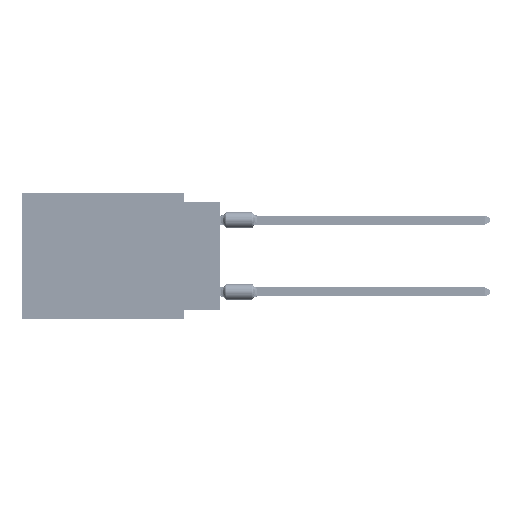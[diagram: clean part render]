
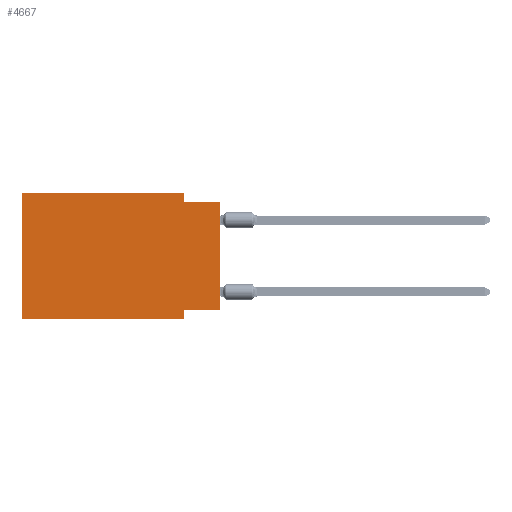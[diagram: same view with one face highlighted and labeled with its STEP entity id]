
A CAD part, left-side view. The second image highlights one B-rep face of the part: STEP entity #4667.
In plain terms, the highlighted planar face has unit normal (-1, 0, 0).
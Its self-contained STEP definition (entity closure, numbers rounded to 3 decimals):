
#9 = ORIENTED_EDGE ( 'NONE', *, *, #9248, .F. ) ;
#774 = CARTESIAN_POINT ( 'NONE',  ( 0., 0., -0.635 ) ) ;
#1195 = ORIENTED_EDGE ( 'NONE', *, *, #63471, .T. ) ;
#1686 = VECTOR ( 'NONE', #52025, 1000. ) ;
#3963 = FACE_OUTER_BOUND ( 'NONE', #36349, .T. ) ;
#4667 = ADVANCED_FACE ( 'NONE', ( #3963 ), #26721, .F. ) ;
#5052 = VECTOR ( 'NONE', #40132, 1000. ) ;
#9248 = EDGE_CURVE ( 'NONE', #35094, #36176, #18670, .T. ) ;
#10494 = CARTESIAN_POINT ( 'NONE',  ( 0., 2.54, 0. ) ) ;
#11138 = VERTEX_POINT ( 'NONE', #43943 ) ;
#11464 = ORIENTED_EDGE ( 'NONE', *, *, #60808, .T. ) ;
#11735 = CARTESIAN_POINT ( 'NONE',  ( 0., 13.97, 0. ) ) ;
#15863 = VECTOR ( 'NONE', #48793, 1000. ) ;
#17369 = CARTESIAN_POINT ( 'NONE',  ( 0., 0., 0. ) ) ;
#18155 = CARTESIAN_POINT ( 'NONE',  ( 0., 2.54, -0.635 ) ) ;
#18670 = LINE ( 'NONE', #774, #35137 ) ;
#19192 = DIRECTION ( 'NONE',  ( 0., 0., -1. ) ) ;
#25318 = LINE ( 'NONE', #36872, #64845 ) ;
#25639 = EDGE_CURVE ( 'NONE', #57394, #62763, #62853, .T. ) ;
#25906 = CARTESIAN_POINT ( 'NONE',  ( 0., 2.54, -8.255 ) ) ;
#26721 = PLANE ( 'NONE',  #33667 ) ;
#26911 = VECTOR ( 'NONE', #45616, 1000. ) ;
#27464 = LINE ( 'NONE', #17369, #5052 ) ;
#29653 = LINE ( 'NONE', #43069, #61893 ) ;
#30845 = ORIENTED_EDGE ( 'NONE', *, *, #61746, .F. ) ;
#33667 = AXIS2_PLACEMENT_3D ( 'NONE', #63989, #68833, #34519 ) ;
#34305 = VECTOR ( 'NONE', #72657, 1000. ) ;
#34427 = LINE ( 'NONE', #40019, #26911 ) ;
#34519 = DIRECTION ( 'NONE',  ( 0., 0., -1. ) ) ;
#35094 = VERTEX_POINT ( 'NONE', #18155 ) ;
#35137 = VECTOR ( 'NONE', #47785, 1000. ) ;
#36176 = VERTEX_POINT ( 'NONE', #60513 ) ;
#36349 = EDGE_LOOP ( 'NONE', ( #11464, #9, #61384, #51755, #50600, #1195, #67252, #30845 ) ) ;
#36872 = CARTESIAN_POINT ( 'NONE',  ( 0., 13.97, -8.89 ) ) ;
#36985 = CARTESIAN_POINT ( 'NONE',  ( 0., 2.54, -8.89 ) ) ;
#37939 = CARTESIAN_POINT ( 'NONE',  ( 0., 0., -8.255 ) ) ;
#40019 = CARTESIAN_POINT ( 'NONE',  ( 0., 13.97, 0. ) ) ;
#40132 = DIRECTION ( 'NONE',  ( 0., 0., 1. ) ) ;
#40844 = CARTESIAN_POINT ( 'NONE',  ( 0., 13.97, 0. ) ) ;
#43069 = CARTESIAN_POINT ( 'NONE',  ( 0., 2.54, 0. ) ) ;
#43462 = CARTESIAN_POINT ( 'NONE',  ( 0., 0., -8.255 ) ) ;
#43943 = CARTESIAN_POINT ( 'NONE',  ( 0., 13.97, -8.89 ) ) ;
#44294 = LINE ( 'NONE', #73377, #34305 ) ;
#45616 = DIRECTION ( 'NONE',  ( 0., 0., 1. ) ) ;
#47785 = DIRECTION ( 'NONE',  ( 0., -1., 0. ) ) ;
#48793 = DIRECTION ( 'NONE',  ( 0., 1., 0. ) ) ;
#50600 = ORIENTED_EDGE ( 'NONE', *, *, #51487, .F. ) ;
#51487 = EDGE_CURVE ( 'NONE', #11138, #57394, #34427, .T. ) ;
#51755 = ORIENTED_EDGE ( 'NONE', *, *, #25639, .F. ) ;
#52025 = DIRECTION ( 'NONE',  ( 0., -1., 0. ) ) ;
#54254 = EDGE_CURVE ( 'NONE', #58826, #66364, #44294, .T. ) ;
#57394 = VERTEX_POINT ( 'NONE', #40844 ) ;
#57398 = EDGE_CURVE ( 'NONE', #62763, #35094, #29653, .T. ) ;
#58826 = VERTEX_POINT ( 'NONE', #25906 ) ;
#59654 = DIRECTION ( 'NONE',  ( 0., -1., 0. ) ) ;
#60513 = CARTESIAN_POINT ( 'NONE',  ( 0., 0., -0.635 ) ) ;
#60808 = EDGE_CURVE ( 'NONE', #61013, #36176, #27464, .T. ) ;
#61013 = VERTEX_POINT ( 'NONE', #43462 ) ;
#61384 = ORIENTED_EDGE ( 'NONE', *, *, #57398, .F. ) ;
#61746 = EDGE_CURVE ( 'NONE', #61013, #58826, #65952, .T. ) ;
#61893 = VECTOR ( 'NONE', #19192, 1000. ) ;
#62763 = VERTEX_POINT ( 'NONE', #10494 ) ;
#62853 = LINE ( 'NONE', #11735, #1686 ) ;
#63471 = EDGE_CURVE ( 'NONE', #11138, #66364, #25318, .T. ) ;
#63989 = CARTESIAN_POINT ( 'NONE',  ( 0., 13.97, 0. ) ) ;
#64845 = VECTOR ( 'NONE', #59654, 1000. ) ;
#65952 = LINE ( 'NONE', #37939, #15863 ) ;
#66364 = VERTEX_POINT ( 'NONE', #36985 ) ;
#67252 = ORIENTED_EDGE ( 'NONE', *, *, #54254, .F. ) ;
#68833 = DIRECTION ( 'NONE',  ( 1., 0., 0. ) ) ;
#72657 = DIRECTION ( 'NONE',  ( 0., 0., -1. ) ) ;
#73377 = CARTESIAN_POINT ( 'NONE',  ( 0., 2.54, -8.89 ) ) ;
